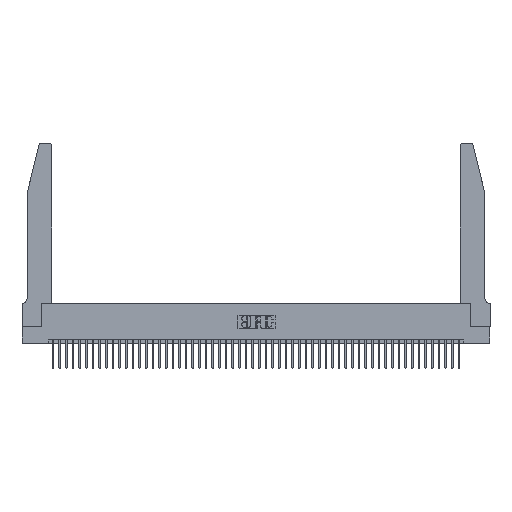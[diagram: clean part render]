
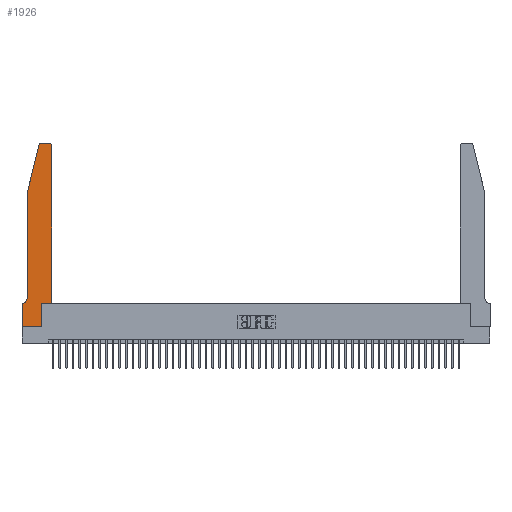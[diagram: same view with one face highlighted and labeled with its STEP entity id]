
A CAD part, top view. The second image highlights one B-rep face of the part: STEP entity #1926.
In plain terms, the highlighted planar face has unit normal (0, 0, 1).
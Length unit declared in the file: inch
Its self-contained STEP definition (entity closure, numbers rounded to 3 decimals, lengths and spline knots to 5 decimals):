
#23 = EDGE_CURVE ( 'NONE', #10429, #43477, #41910, .T. ) ;
#554 = CARTESIAN_POINT ( 'NONE',  ( 0.284, 2.75, 0.37 ) ) ;
#1336 = CIRCLE ( 'NONE', #7503, 0.03 ) ;
#1926 = ADVANCED_FACE ( 'NONE', ( #5011 ), #26076, .T. ) ;
#2330 = EDGE_CURVE ( 'NONE', #23322, #29582, #44132, .T. ) ;
#2504 = DIRECTION ( 'NONE',  ( -1., 0., 0. ) ) ;
#2684 = CARTESIAN_POINT ( 'NONE',  ( 0.4505, 0.35, 0.37 ) ) ;
#5011 = FACE_OUTER_BOUND ( 'NONE', #32216, .T. ) ;
#5807 = VECTOR ( 'NONE', #16905, 39.37008 ) ;
#6143 = CARTESIAN_POINT ( 'NONE',  ( 0.0055, 0.42, 0.37 ) ) ;
#6976 = ORIENTED_EDGE ( 'NONE', *, *, #33844, .T. ) ;
#7503 = AXIS2_PLACEMENT_3D ( 'NONE', #38871, #35121, #46919 ) ;
#7710 = ORIENTED_EDGE ( 'NONE', *, *, #23, .T. ) ;
#7898 = VECTOR ( 'NONE', #10853, 39.37008 ) ;
#8040 = CARTESIAN_POINT ( 'NONE',  ( 0.4505, 0.35, 0.37 ) ) ;
#8490 = ORIENTED_EDGE ( 'NONE', *, *, #44502, .T. ) ;
#8902 = EDGE_CURVE ( 'NONE', #41120, #15628, #29966, .T. ) ;
#9720 = CARTESIAN_POINT ( 'NONE',  ( 0., 0., 0.37 ) ) ;
#10218 = CARTESIAN_POINT ( 'NONE',  ( 0., 0.35, 0.37 ) ) ;
#10429 = VERTEX_POINT ( 'NONE', #40212 ) ;
#10554 = DIRECTION ( 'NONE',  ( 0., 0., 1. ) ) ;
#10575 = CIRCLE ( 'NONE', #47205, 0.07 ) ;
#10853 = DIRECTION ( 'NONE',  ( -1., 0., 0. ) ) ;
#10945 = ORIENTED_EDGE ( 'NONE', *, *, #20956, .T. ) ;
#11102 = DIRECTION ( 'NONE',  ( 0., 0., 1. ) ) ;
#11676 = CARTESIAN_POINT ( 'NONE',  ( 0.2865, 0.35, 0.37 ) ) ;
#12005 = ORIENTED_EDGE ( 'NONE', *, *, #8902, .T. ) ;
#12982 = CARTESIAN_POINT ( 'NONE',  ( 0.0755, 2., 0.37 ) ) ;
#13928 = VECTOR ( 'NONE', #22706, 39.37008 ) ;
#13953 = VERTEX_POINT ( 'NONE', #9720 ) ;
#14776 = VERTEX_POINT ( 'NONE', #18826 ) ;
#15401 = EDGE_CURVE ( 'NONE', #29582, #18985, #34696, .T. ) ;
#15628 = VERTEX_POINT ( 'NONE', #554 ) ;
#16633 = VECTOR ( 'NONE', #27558, 39.37008 ) ;
#16905 = DIRECTION ( 'NONE',  ( 0., -1., 0. ) ) ;
#18041 = ORIENTED_EDGE ( 'NONE', *, *, #45959, .T. ) ;
#18397 = DIRECTION ( 'NONE',  ( 1., 0., 0. ) ) ;
#18531 = DIRECTION ( 'NONE',  ( -0.239, -0.971, 0. ) ) ;
#18595 = LINE ( 'NONE', #2684, #19765 ) ;
#18826 = CARTESIAN_POINT ( 'NONE',  ( 0.4505, 2.72, 0.37 ) ) ;
#18985 = VERTEX_POINT ( 'NONE', #8040 ) ;
#19321 = CIRCLE ( 'NONE', #48581, 0.03 ) ;
#19765 = VECTOR ( 'NONE', #34185, 39.37008 ) ;
#20767 = VECTOR ( 'NONE', #18531, 39.37008 ) ;
#20956 = EDGE_CURVE ( 'NONE', #24744, #13953, #29972, .T. ) ;
#21061 = ORIENTED_EDGE ( 'NONE', *, *, #46609, .T. ) ;
#21071 = CARTESIAN_POINT ( 'NONE',  ( 0.2865, 0., 0.37 ) ) ;
#22706 = DIRECTION ( 'NONE',  ( 1., 0., 0. ) ) ;
#23322 = VERTEX_POINT ( 'NONE', #21071 ) ;
#24744 = VERTEX_POINT ( 'NONE', #32752 ) ;
#25443 = VERTEX_POINT ( 'NONE', #46657 ) ;
#25803 = VERTEX_POINT ( 'NONE', #28897 ) ;
#26025 = ORIENTED_EDGE ( 'NONE', *, *, #38539, .T. ) ;
#26076 = PLANE ( 'NONE',  #43896 ) ;
#26800 = CARTESIAN_POINT ( 'NONE',  ( 0.4205, 2.72, 0.37 ) ) ;
#27304 = VECTOR ( 'NONE', #36053, 39.37008 ) ;
#27512 = DIRECTION ( 'NONE',  ( 0., -1., 0. ) ) ;
#27558 = DIRECTION ( 'NONE',  ( 0., 1., 0. ) ) ;
#28375 = EDGE_CURVE ( 'NONE', #14776, #41120, #19321, .T. ) ;
#28897 = CARTESIAN_POINT ( 'NONE',  ( 0.25487, 2.72718, 0.37 ) ) ;
#29582 = VERTEX_POINT ( 'NONE', #11676 ) ;
#29951 = LINE ( 'NONE', #34083, #20767 ) ;
#29966 = LINE ( 'NONE', #34247, #7898 ) ;
#29972 = LINE ( 'NONE', #39797, #49543 ) ;
#30743 = ORIENTED_EDGE ( 'NONE', *, *, #2330, .T. ) ;
#30959 = DIRECTION ( 'NONE',  ( 0., 0., -1. ) ) ;
#30983 = EDGE_CURVE ( 'NONE', #15628, #25803, #1336, .T. ) ;
#32216 = EDGE_LOOP ( 'NONE', ( #12005, #43810, #18041, #7710, #8490, #26025, #10945, #6976, #30743, #33039, #21061, #33203 ) ) ;
#32644 = CARTESIAN_POINT ( 'NONE',  ( 0., 0., 0.37 ) ) ;
#32752 = CARTESIAN_POINT ( 'NONE',  ( 0., 0.35, 0.37 ) ) ;
#33039 = ORIENTED_EDGE ( 'NONE', *, *, #15401, .T. ) ;
#33203 = ORIENTED_EDGE ( 'NONE', *, *, #28375, .T. ) ;
#33844 = EDGE_CURVE ( 'NONE', #13953, #23322, #37717, .T. ) ;
#34083 = CARTESIAN_POINT ( 'NONE',  ( 0.0755, 2., 0.37 ) ) ;
#34185 = DIRECTION ( 'NONE',  ( 0., 1., 0. ) ) ;
#34247 = CARTESIAN_POINT ( 'NONE',  ( 0.2605, 2.75, 0.37 ) ) ;
#34641 = CARTESIAN_POINT ( 'NONE',  ( 0.4505, 0.35, 0.37 ) ) ;
#34696 = LINE ( 'NONE', #34641, #13928 ) ;
#35121 = DIRECTION ( 'NONE',  ( 0., 0., 1. ) ) ;
#36053 = DIRECTION ( 'NONE',  ( 1., 0., 0. ) ) ;
#37717 = LINE ( 'NONE', #32644, #27304 ) ;
#37755 = CARTESIAN_POINT ( 'NONE',  ( 0.4205, 2.75, 0.37 ) ) ;
#38185 = CARTESIAN_POINT ( 'NONE',  ( 0.0755, 0.35, 0.37 ) ) ;
#38539 = EDGE_CURVE ( 'NONE', #25443, #24744, #43359, .T. ) ;
#38871 = CARTESIAN_POINT ( 'NONE',  ( 0.284, 2.72, 0.37 ) ) ;
#39797 = CARTESIAN_POINT ( 'NONE',  ( 0., 0., 0.37 ) ) ;
#40212 = CARTESIAN_POINT ( 'NONE',  ( 0.0755, 2., 0.37 ) ) ;
#41120 = VERTEX_POINT ( 'NONE', #37755 ) ;
#41910 = LINE ( 'NONE', #12982, #5807 ) ;
#42571 = DIRECTION ( 'NONE',  ( -1., 0., 0. ) ) ;
#42723 = CARTESIAN_POINT ( 'NONE',  ( 0.2865, 0.35, 0.37 ) ) ;
#43359 = LINE ( 'NONE', #38185, #46457 ) ;
#43477 = VERTEX_POINT ( 'NONE', #46415 ) ;
#43810 = ORIENTED_EDGE ( 'NONE', *, *, #30983, .T. ) ;
#43896 = AXIS2_PLACEMENT_3D ( 'NONE', #10218, #10554, #18397 ) ;
#44132 = LINE ( 'NONE', #42723, #16633 ) ;
#44502 = EDGE_CURVE ( 'NONE', #43477, #25443, #10575, .T. ) ;
#45959 = EDGE_CURVE ( 'NONE', #25803, #10429, #29951, .T. ) ;
#46415 = CARTESIAN_POINT ( 'NONE',  ( 0.0755, 0.42, 0.37 ) ) ;
#46452 = DIRECTION ( 'NONE',  ( 1., 0., 0. ) ) ;
#46457 = VECTOR ( 'NONE', #42571, 39.37008 ) ;
#46609 = EDGE_CURVE ( 'NONE', #18985, #14776, #18595, .T. ) ;
#46657 = CARTESIAN_POINT ( 'NONE',  ( 0.0055, 0.35, 0.37 ) ) ;
#46919 = DIRECTION ( 'NONE',  ( 1., 0., 0. ) ) ;
#47205 = AXIS2_PLACEMENT_3D ( 'NONE', #6143, #30959, #2504 ) ;
#48581 = AXIS2_PLACEMENT_3D ( 'NONE', #26800, #11102, #46452 ) ;
#49543 = VECTOR ( 'NONE', #27512, 39.37008 ) ;
